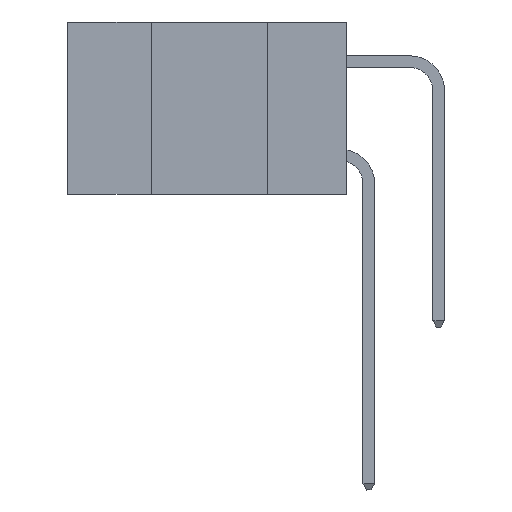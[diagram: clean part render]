
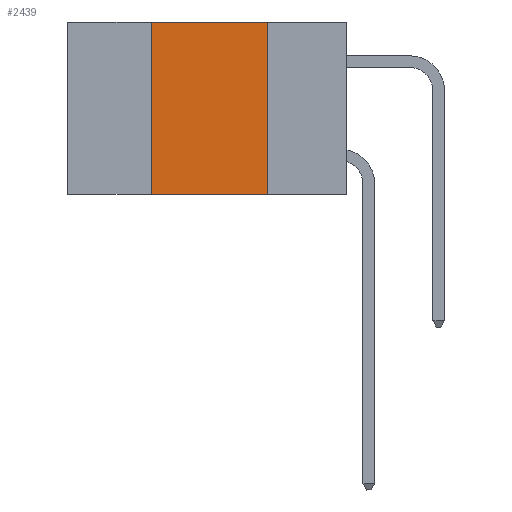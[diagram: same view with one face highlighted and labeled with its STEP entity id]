
A CAD part, left-side view. The second image highlights one B-rep face of the part: STEP entity #2439.
In plain terms, the highlighted planar face has unit normal (-1, 0, 0).
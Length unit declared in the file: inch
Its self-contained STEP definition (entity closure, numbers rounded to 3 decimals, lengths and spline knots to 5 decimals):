
#416 = LINE ( 'NONE', #1570, #1709 ) ;
#1303 = LINE ( 'NONE', #12145, #11768 ) ;
#1518 = DIRECTION ( 'NONE',  ( 0., -1., 0. ) ) ;
#1570 = CARTESIAN_POINT ( 'NONE',  ( 0., 0.6, 0. ) ) ;
#1648 = LINE ( 'NONE', #5543, #6225 ) ;
#1682 = ORIENTED_EDGE ( 'NONE', *, *, #14480, .F. ) ;
#1709 = VECTOR ( 'NONE', #1518, 39.37008 ) ;
#1985 = DIRECTION ( 'NONE',  ( 0., 0., 1. ) ) ;
#2107 = DIRECTION ( 'NONE',  ( 0., 0., -1. ) ) ;
#2137 = ORIENTED_EDGE ( 'NONE', *, *, #3739, .F. ) ;
#2439 = ADVANCED_FACE ( 'NONE', ( #11652 ), #3644, .F. ) ;
#2572 = CARTESIAN_POINT ( 'NONE',  ( 0., 0.17, 0. ) ) ;
#3636 = CARTESIAN_POINT ( 'NONE',  ( 0., 0.42, 0. ) ) ;
#3644 = PLANE ( 'NONE',  #4128 ) ;
#3739 = EDGE_CURVE ( 'NONE', #13057, #4856, #416, .T. ) ;
#4128 = AXIS2_PLACEMENT_3D ( 'NONE', #8125, #6950, #15253 ) ;
#4236 = CARTESIAN_POINT ( 'NONE',  ( 0., 0.42, -0.37 ) ) ;
#4856 = VERTEX_POINT ( 'NONE', #2572 ) ;
#5002 = VECTOR ( 'NONE', #1985, 39.37008 ) ;
#5543 = CARTESIAN_POINT ( 'NONE',  ( 0., 0.17, 0. ) ) ;
#6225 = VECTOR ( 'NONE', #2107, 39.37008 ) ;
#6705 = ORIENTED_EDGE ( 'NONE', *, *, #11911, .F. ) ;
#6950 = DIRECTION ( 'NONE',  ( 1., 0., 0. ) ) ;
#7051 = VERTEX_POINT ( 'NONE', #11321 ) ;
#7871 = ORIENTED_EDGE ( 'NONE', *, *, #13219, .T. ) ;
#8116 = VERTEX_POINT ( 'NONE', #4236 ) ;
#8125 = CARTESIAN_POINT ( 'NONE',  ( 0., 0.6, 0. ) ) ;
#8350 = CARTESIAN_POINT ( 'NONE',  ( 0., 0.42, 0. ) ) ;
#9214 = LINE ( 'NONE', #3636, #5002 ) ;
#11321 = CARTESIAN_POINT ( 'NONE',  ( 0., 0.17, -0.37 ) ) ;
#11652 = FACE_OUTER_BOUND ( 'NONE', #14972, .T. ) ;
#11768 = VECTOR ( 'NONE', #13244, 39.37008 ) ;
#11911 = EDGE_CURVE ( 'NONE', #8116, #13057, #9214, .T. ) ;
#12145 = CARTESIAN_POINT ( 'NONE',  ( 0., 0.6, -0.37 ) ) ;
#13057 = VERTEX_POINT ( 'NONE', #8350 ) ;
#13219 = EDGE_CURVE ( 'NONE', #8116, #7051, #1303, .T. ) ;
#13244 = DIRECTION ( 'NONE',  ( 0., -1., 0. ) ) ;
#14480 = EDGE_CURVE ( 'NONE', #4856, #7051, #1648, .T. ) ;
#14972 = EDGE_LOOP ( 'NONE', ( #1682, #2137, #6705, #7871 ) ) ;
#15253 = DIRECTION ( 'NONE',  ( 0., 0., -1. ) ) ;
